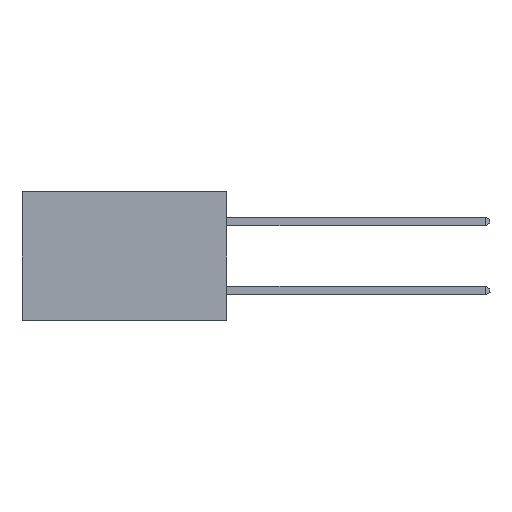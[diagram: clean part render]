
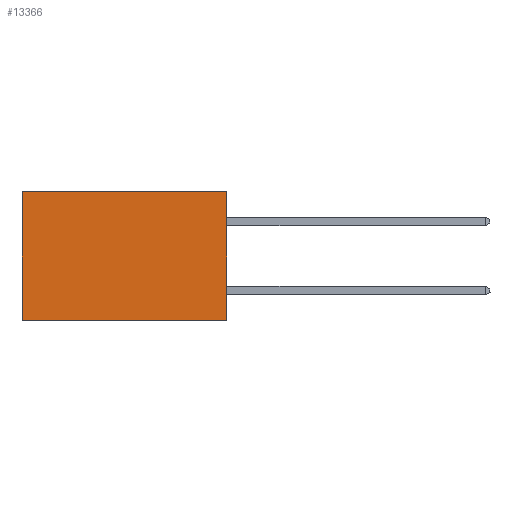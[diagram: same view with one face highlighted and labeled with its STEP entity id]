
A CAD part, left-side view. The second image highlights one B-rep face of the part: STEP entity #13366.
In plain terms, the highlighted planar face has unit normal (-1, 0, 0).
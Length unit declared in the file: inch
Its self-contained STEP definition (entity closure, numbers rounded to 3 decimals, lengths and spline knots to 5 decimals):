
#481 = FACE_OUTER_BOUND ( 'NONE', #6710, .T. ) ;
#1571 = EDGE_CURVE ( 'NONE', #13142, #5156, #1897, .T. ) ;
#1709 = EDGE_CURVE ( 'NONE', #5156, #4819, #3889, .T. ) ;
#1897 = LINE ( 'NONE', #12390, #6203 ) ;
#2228 = LINE ( 'NONE', #13513, #19274 ) ;
#2403 = CARTESIAN_POINT ( 'NONE',  ( 0.277, 0.59, -0.37 ) ) ;
#2701 = DIRECTION ( 'NONE',  ( 0., 0., -1. ) ) ;
#3189 = PLANE ( 'NONE',  #14046 ) ;
#3303 = VECTOR ( 'NONE', #5673, 39.37008 ) ;
#3363 = DIRECTION ( 'NONE',  ( 0., 1., 0. ) ) ;
#3889 = LINE ( 'NONE', #2403, #3303 ) ;
#4819 = VERTEX_POINT ( 'NONE', #7430 ) ;
#5060 = CARTESIAN_POINT ( 'NONE',  ( 0.277, 0., -0.37 ) ) ;
#5156 = VERTEX_POINT ( 'NONE', #18470 ) ;
#5673 = DIRECTION ( 'NONE',  ( 0., 0., -1. ) ) ;
#6203 = VECTOR ( 'NONE', #3363, 39.37008 ) ;
#6344 = CARTESIAN_POINT ( 'NONE',  ( 0.277, 0., -0.37 ) ) ;
#6710 = EDGE_LOOP ( 'NONE', ( #17868, #15656, #7993, #11961 ) ) ;
#6920 = DIRECTION ( 'NONE',  ( 1., 0., 0. ) ) ;
#7430 = CARTESIAN_POINT ( 'NONE',  ( 0.277, 0.59, -0.37 ) ) ;
#7993 = ORIENTED_EDGE ( 'NONE', *, *, #18517, .F. ) ;
#11865 = LINE ( 'NONE', #6344, #15028 ) ;
#11961 = ORIENTED_EDGE ( 'NONE', *, *, #1571, .T. ) ;
#12390 = CARTESIAN_POINT ( 'NONE',  ( 0.277, 0., 0. ) ) ;
#12456 = EDGE_CURVE ( 'NONE', #13683, #4819, #2228, .T. ) ;
#13142 = VERTEX_POINT ( 'NONE', #20719 ) ;
#13366 = ADVANCED_FACE ( 'NONE', ( #481 ), #3189, .F. ) ;
#13513 = CARTESIAN_POINT ( 'NONE',  ( 0.277, 0., -0.37 ) ) ;
#13683 = VERTEX_POINT ( 'NONE', #18434 ) ;
#14046 = AXIS2_PLACEMENT_3D ( 'NONE', #5060, #6920, #19547 ) ;
#15028 = VECTOR ( 'NONE', #2701, 39.37008 ) ;
#15369 = DIRECTION ( 'NONE',  ( 0., 1., 0. ) ) ;
#15656 = ORIENTED_EDGE ( 'NONE', *, *, #12456, .F. ) ;
#17868 = ORIENTED_EDGE ( 'NONE', *, *, #1709, .T. ) ;
#18434 = CARTESIAN_POINT ( 'NONE',  ( 0.277, 0., -0.37 ) ) ;
#18470 = CARTESIAN_POINT ( 'NONE',  ( 0.277, 0.59, 0. ) ) ;
#18517 = EDGE_CURVE ( 'NONE', #13142, #13683, #11865, .T. ) ;
#19274 = VECTOR ( 'NONE', #15369, 39.37008 ) ;
#19547 = DIRECTION ( 'NONE',  ( 0., 0., -1. ) ) ;
#20719 = CARTESIAN_POINT ( 'NONE',  ( 0.277, 0., 0. ) ) ;
